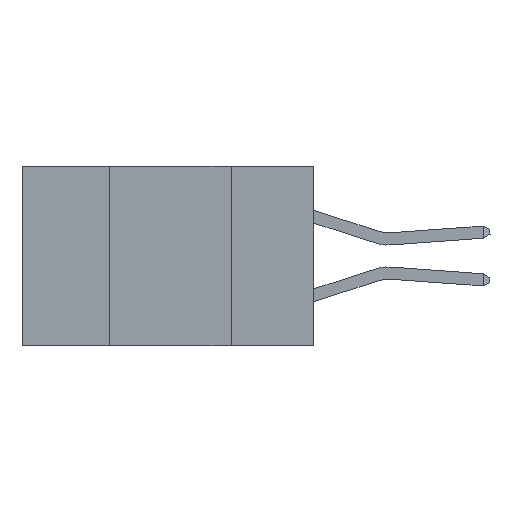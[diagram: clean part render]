
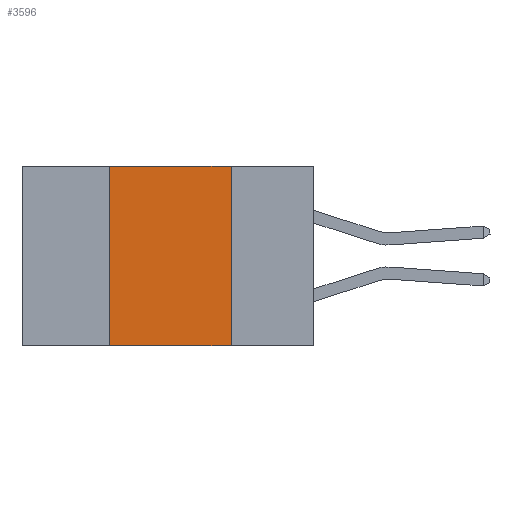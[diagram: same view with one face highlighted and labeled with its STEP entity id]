
A CAD part, left-side view. The second image highlights one B-rep face of the part: STEP entity #3596.
In plain terms, the highlighted planar face has unit normal (-1, 0, 0).
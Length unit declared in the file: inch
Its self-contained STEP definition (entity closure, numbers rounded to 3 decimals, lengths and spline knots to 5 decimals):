
#131 = CARTESIAN_POINT ( 'NONE',  ( 0., 0.17, -0.37 ) ) ;
#445 = DIRECTION ( 'NONE',  ( 0., 0., -1. ) ) ;
#519 = VERTEX_POINT ( 'NONE', #2846 ) ;
#699 = VECTOR ( 'NONE', #9149, 39.37008 ) ;
#713 = CARTESIAN_POINT ( 'NONE',  ( 0., 0.17, 0. ) ) ;
#1138 = ORIENTED_EDGE ( 'NONE', *, *, #1175, .T. ) ;
#1175 = EDGE_CURVE ( 'NONE', #10099, #1815, #10637, .T. ) ;
#1328 = CARTESIAN_POINT ( 'NONE',  ( 0., 0.6, 0. ) ) ;
#1434 = PLANE ( 'NONE',  #9053 ) ;
#1695 = LINE ( 'NONE', #11314, #7617 ) ;
#1815 = VERTEX_POINT ( 'NONE', #131 ) ;
#2640 = DIRECTION ( 'NONE',  ( 0., -1., 0. ) ) ;
#2846 = CARTESIAN_POINT ( 'NONE',  ( 0., 0.17, 0. ) ) ;
#2866 = EDGE_CURVE ( 'NONE', #2972, #519, #1695, .T. ) ;
#2889 = ORIENTED_EDGE ( 'NONE', *, *, #7789, .F. ) ;
#2972 = VERTEX_POINT ( 'NONE', #3649 ) ;
#3596 = ADVANCED_FACE ( 'NONE', ( #9401 ), #1434, .F. ) ;
#3649 = CARTESIAN_POINT ( 'NONE',  ( 0., 0.42, 0. ) ) ;
#4082 = LINE ( 'NONE', #713, #10334 ) ;
#4247 = DIRECTION ( 'NONE',  ( 0., 0., -1. ) ) ;
#4713 = LINE ( 'NONE', #8169, #699 ) ;
#5932 = VECTOR ( 'NONE', #2640, 39.37008 ) ;
#6298 = EDGE_CURVE ( 'NONE', #519, #1815, #4082, .T. ) ;
#6344 = ORIENTED_EDGE ( 'NONE', *, *, #2866, .F. ) ;
#7018 = CARTESIAN_POINT ( 'NONE',  ( 0., 0.42, -0.37 ) ) ;
#7617 = VECTOR ( 'NONE', #9501, 39.37008 ) ;
#7789 = EDGE_CURVE ( 'NONE', #10099, #2972, #4713, .T. ) ;
#7869 = ORIENTED_EDGE ( 'NONE', *, *, #6298, .F. ) ;
#8169 = CARTESIAN_POINT ( 'NONE',  ( 0., 0.42, 0. ) ) ;
#8538 = DIRECTION ( 'NONE',  ( 1., 0., 0. ) ) ;
#8829 = CARTESIAN_POINT ( 'NONE',  ( 0., 0.6, -0.37 ) ) ;
#9053 = AXIS2_PLACEMENT_3D ( 'NONE', #1328, #8538, #445 ) ;
#9149 = DIRECTION ( 'NONE',  ( 0., 0., 1. ) ) ;
#9401 = FACE_OUTER_BOUND ( 'NONE', #10177, .T. ) ;
#9501 = DIRECTION ( 'NONE',  ( 0., -1., 0. ) ) ;
#10099 = VERTEX_POINT ( 'NONE', #7018 ) ;
#10177 = EDGE_LOOP ( 'NONE', ( #7869, #6344, #2889, #1138 ) ) ;
#10334 = VECTOR ( 'NONE', #4247, 39.37008 ) ;
#10637 = LINE ( 'NONE', #8829, #5932 ) ;
#11314 = CARTESIAN_POINT ( 'NONE',  ( 0., 0.6, 0. ) ) ;
